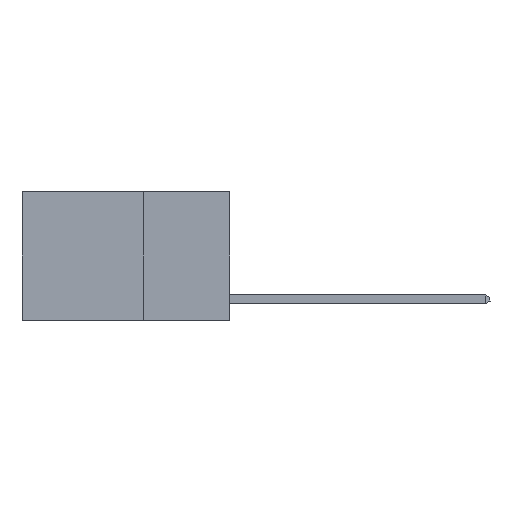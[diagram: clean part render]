
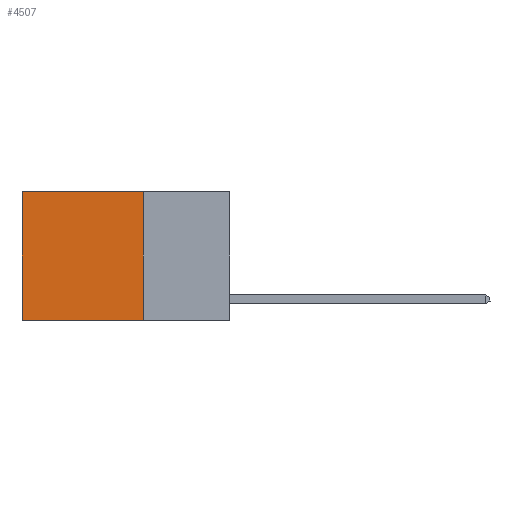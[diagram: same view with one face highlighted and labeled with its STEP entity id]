
A CAD part, left-side view. The second image highlights one B-rep face of the part: STEP entity #4507.
In plain terms, the highlighted planar face has unit normal (-1, 0, 0).
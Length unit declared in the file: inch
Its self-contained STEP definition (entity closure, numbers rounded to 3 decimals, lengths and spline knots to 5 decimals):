
#319 = LINE ( 'NONE', #10005, #9362 ) ;
#1040 = ORIENTED_EDGE ( 'NONE', *, *, #10556, .F. ) ;
#1824 = DIRECTION ( 'NONE',  ( 0., 0., -1. ) ) ;
#3497 = AXIS2_PLACEMENT_3D ( 'NONE', #7339, #8976, #20157 ) ;
#3498 = VERTEX_POINT ( 'NONE', #8243 ) ;
#4028 = FACE_OUTER_BOUND ( 'NONE', #4073, .T. ) ;
#4073 = EDGE_LOOP ( 'NONE', ( #13957, #1040, #16948, #11299 ) ) ;
#4507 = ADVANCED_FACE ( 'NONE', ( #4028 ), #16987, .F. ) ;
#4598 = CARTESIAN_POINT ( 'NONE',  ( 0.2625, 0.6, 0. ) ) ;
#5153 = CARTESIAN_POINT ( 'NONE',  ( 0.2625, 0.6, 0. ) ) ;
#6437 = DIRECTION ( 'NONE',  ( 0., 1., 0. ) ) ;
#6823 = VECTOR ( 'NONE', #6437, 39.37008 ) ;
#7339 = CARTESIAN_POINT ( 'NONE',  ( 0.2625, 0.25, 0. ) ) ;
#7929 = VECTOR ( 'NONE', #14269, 39.37008 ) ;
#8243 = CARTESIAN_POINT ( 'NONE',  ( 0.2625, 0.25, -0.37 ) ) ;
#8976 = DIRECTION ( 'NONE',  ( 1., 0., 0. ) ) ;
#9362 = VECTOR ( 'NONE', #11621, 39.37008 ) ;
#9851 = CARTESIAN_POINT ( 'NONE',  ( 0.2625, 0.25, 0. ) ) ;
#10005 = CARTESIAN_POINT ( 'NONE',  ( 0.2625, 0.25, -0.37 ) ) ;
#10079 = VERTEX_POINT ( 'NONE', #19902 ) ;
#10489 = EDGE_CURVE ( 'NONE', #10527, #3498, #14165, .T. ) ;
#10527 = VERTEX_POINT ( 'NONE', #14695 ) ;
#10556 = EDGE_CURVE ( 'NONE', #3498, #10079, #319, .T. ) ;
#11019 = EDGE_CURVE ( 'NONE', #10527, #13751, #20588, .T. ) ;
#11256 = CARTESIAN_POINT ( 'NONE',  ( 0.2625, 0.25, 0. ) ) ;
#11299 = ORIENTED_EDGE ( 'NONE', *, *, #11019, .T. ) ;
#11621 = DIRECTION ( 'NONE',  ( 0., 1., 0. ) ) ;
#12237 = LINE ( 'NONE', #4598, #7929 ) ;
#13680 = VECTOR ( 'NONE', #1824, 39.37008 ) ;
#13751 = VERTEX_POINT ( 'NONE', #5153 ) ;
#13957 = ORIENTED_EDGE ( 'NONE', *, *, #19361, .T. ) ;
#14165 = LINE ( 'NONE', #9851, #13680 ) ;
#14269 = DIRECTION ( 'NONE',  ( 0., 0., -1. ) ) ;
#14695 = CARTESIAN_POINT ( 'NONE',  ( 0.2625, 0.25, 0. ) ) ;
#16948 = ORIENTED_EDGE ( 'NONE', *, *, #10489, .F. ) ;
#16987 = PLANE ( 'NONE',  #3497 ) ;
#19361 = EDGE_CURVE ( 'NONE', #13751, #10079, #12237, .T. ) ;
#19902 = CARTESIAN_POINT ( 'NONE',  ( 0.2625, 0.6, -0.37 ) ) ;
#20157 = DIRECTION ( 'NONE',  ( 0., 0., -1. ) ) ;
#20588 = LINE ( 'NONE', #11256, #6823 ) ;
